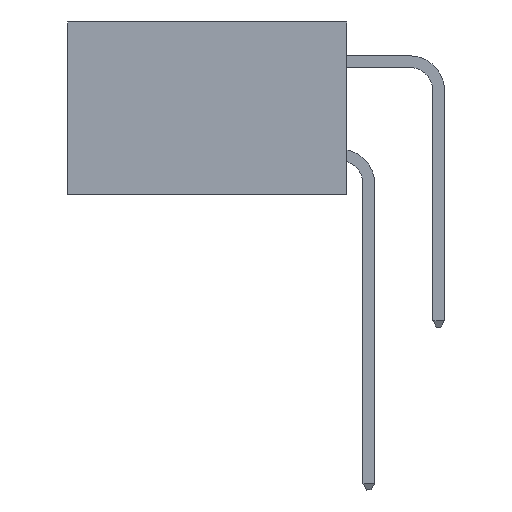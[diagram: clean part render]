
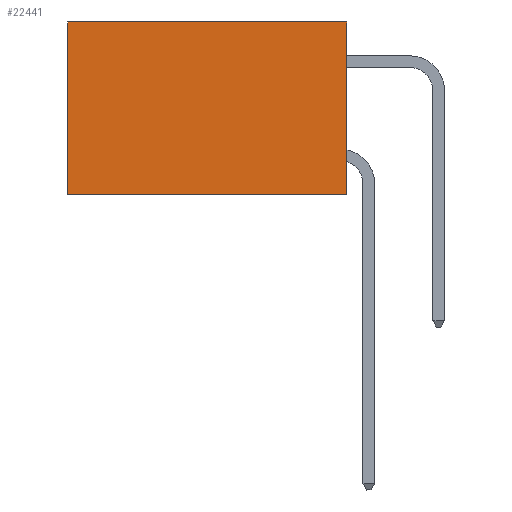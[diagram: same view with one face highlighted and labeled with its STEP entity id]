
A CAD part, left-side view. The second image highlights one B-rep face of the part: STEP entity #22441.
In plain terms, the highlighted planar face has unit normal (-1, 0, 0).
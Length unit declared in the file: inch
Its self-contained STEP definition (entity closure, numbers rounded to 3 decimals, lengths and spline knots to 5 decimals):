
#225 = VECTOR ( 'NONE', #15979, 39.37008 ) ;
#2705 = EDGE_CURVE ( 'NONE', #38268, #13283, #5842, .T. ) ;
#3909 = LINE ( 'NONE', #21126, #9185 ) ;
#4501 = CARTESIAN_POINT ( 'NONE',  ( 0.2875, 0., 0. ) ) ;
#4895 = VECTOR ( 'NONE', #15444, 39.37008 ) ;
#5842 = LINE ( 'NONE', #10413, #4895 ) ;
#6769 = AXIS2_PLACEMENT_3D ( 'NONE', #4501, #7604, #28706 ) ;
#7035 = ORIENTED_EDGE ( 'NONE', *, *, #10796, .F. ) ;
#7604 = DIRECTION ( 'NONE',  ( 1., 0., 0. ) ) ;
#9054 = EDGE_CURVE ( 'NONE', #26856, #33540, #15545, .T. ) ;
#9185 = VECTOR ( 'NONE', #33043, 39.37008 ) ;
#9951 = CARTESIAN_POINT ( 'NONE',  ( 0.2875, 0.6, 0. ) ) ;
#10413 = CARTESIAN_POINT ( 'NONE',  ( 0.2875, 0., 0. ) ) ;
#10796 = EDGE_CURVE ( 'NONE', #13283, #33540, #3909, .T. ) ;
#11574 = VECTOR ( 'NONE', #22113, 39.37008 ) ;
#12532 = LINE ( 'NONE', #36870, #11574 ) ;
#13283 = VERTEX_POINT ( 'NONE', #22553 ) ;
#15444 = DIRECTION ( 'NONE',  ( 0., 0., -1. ) ) ;
#15545 = LINE ( 'NONE', #9951, #225 ) ;
#15979 = DIRECTION ( 'NONE',  ( 0., 0., -1. ) ) ;
#18245 = ORIENTED_EDGE ( 'NONE', *, *, #9054, .T. ) ;
#21126 = CARTESIAN_POINT ( 'NONE',  ( 0.2875, 0., -0.37 ) ) ;
#22113 = DIRECTION ( 'NONE',  ( 0., 1., 0. ) ) ;
#22441 = ADVANCED_FACE ( 'NONE', ( #35979 ), #25703, .F. ) ;
#22553 = CARTESIAN_POINT ( 'NONE',  ( 0.2875, 0., -0.37 ) ) ;
#23550 = EDGE_CURVE ( 'NONE', #38268, #26856, #12532, .T. ) ;
#25385 = CARTESIAN_POINT ( 'NONE',  ( 0.2875, 0., 0. ) ) ;
#25703 = PLANE ( 'NONE',  #6769 ) ;
#26856 = VERTEX_POINT ( 'NONE', #36588 ) ;
#27034 = CARTESIAN_POINT ( 'NONE',  ( 0.2875, 0.6, -0.37 ) ) ;
#27220 = ORIENTED_EDGE ( 'NONE', *, *, #23550, .T. ) ;
#28706 = DIRECTION ( 'NONE',  ( 0., 0., -1. ) ) ;
#30811 = EDGE_LOOP ( 'NONE', ( #18245, #7035, #36637, #27220 ) ) ;
#33043 = DIRECTION ( 'NONE',  ( 0., 1., 0. ) ) ;
#33540 = VERTEX_POINT ( 'NONE', #27034 ) ;
#35979 = FACE_OUTER_BOUND ( 'NONE', #30811, .T. ) ;
#36588 = CARTESIAN_POINT ( 'NONE',  ( 0.2875, 0.6, 0. ) ) ;
#36637 = ORIENTED_EDGE ( 'NONE', *, *, #2705, .F. ) ;
#36870 = CARTESIAN_POINT ( 'NONE',  ( 0.2875, 0., 0. ) ) ;
#38268 = VERTEX_POINT ( 'NONE', #25385 ) ;
